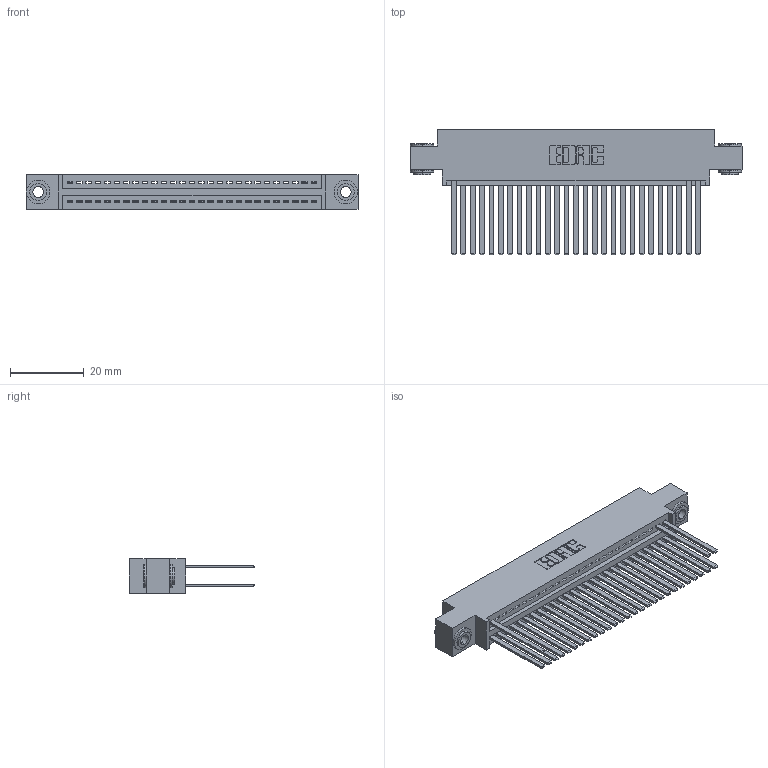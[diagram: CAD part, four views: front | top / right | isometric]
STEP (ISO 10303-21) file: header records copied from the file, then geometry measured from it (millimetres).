
FILE_DESCRIPTION (( 'STEP AP203' ), '1' );
FILE_NAME ('345-054-544-803.STEP', '2018-09-24T00:24:19', ( '' ), ( '' ), 'SwSTEP 2.0', 'SolidWorks 2016', '' );
FILE_SCHEMA (( 'CONFIG_CONTROL_DESIGN' ));
Length unit declared in the file: inch
Products named in the file (4): 345-250-002_345-250-002-102; 345-054-544-803; 345 Part_0.170 Offset - 0.156 Dia-TH; 345-292-001_345-293-144
Assembly tree (33 placements, depth 2):
  345-054-544-803
    345 Part_0.170 Offset - 0.156 Dia-TH
    345-292-001_345-293-144  x30
    345-250-002_345-250-002-102  x2
Bounding box: 89.79 x 33.96 x 9.4 mm (x, y, z)
Volume: 8693.2 mm3; surface area: 12915.1 mm2
Topology: 33 solids, 33 shells, 1680 faces, 5007 edges, 3294 vertices
Faces by surface type: plane 1132, cylinder 540, cone 8
Entity records: 23034 total; most frequent: CARTESIAN_POINT 3955, ORIENTED_EDGE 3906, DIRECTION 3507, EDGE_CURVE 1953, LINE 1693, VECTOR 1693, VERTEX_POINT 1298, AXIS2_PLACEMENT_3D 907
